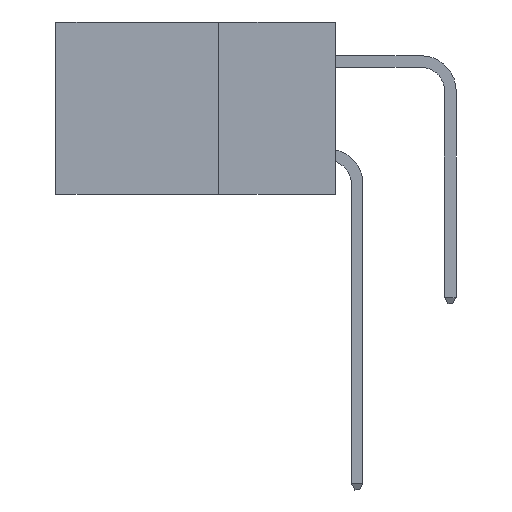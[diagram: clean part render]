
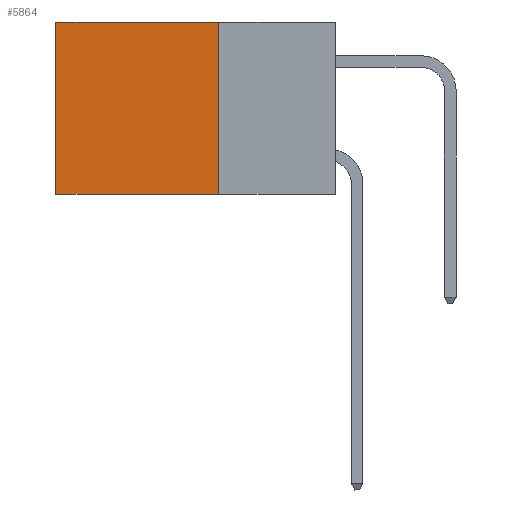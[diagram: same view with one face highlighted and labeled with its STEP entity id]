
A CAD part, left-side view. The second image highlights one B-rep face of the part: STEP entity #5864.
In plain terms, the highlighted planar face has unit normal (-1, 0, 0).
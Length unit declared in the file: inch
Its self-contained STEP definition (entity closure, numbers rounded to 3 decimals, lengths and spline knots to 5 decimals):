
#915 = VERTEX_POINT ( 'NONE', #24425 ) ;
#1086 = EDGE_CURVE ( 'NONE', #12607, #10471, #10237, .T. ) ;
#1834 = EDGE_CURVE ( 'NONE', #25764, #915, #17118, .T. ) ;
#2203 = DIRECTION ( 'NONE',  ( 0., 0., -1. ) ) ;
#3482 = CARTESIAN_POINT ( 'NONE',  ( 0.2875, 0.25, -0.37 ) ) ;
#3589 = VECTOR ( 'NONE', #23332, 39.37008 ) ;
#5864 = ADVANCED_FACE ( 'NONE', ( #30826 ), #12441, .F. ) ;
#6707 = DIRECTION ( 'NONE',  ( 0., 1., 0. ) ) ;
#7108 = VECTOR ( 'NONE', #23282, 39.37008 ) ;
#7812 = LINE ( 'NONE', #18786, #24448 ) ;
#9727 = CARTESIAN_POINT ( 'NONE',  ( 0.2875, 0.25, 0. ) ) ;
#9738 = CARTESIAN_POINT ( 'NONE',  ( 0.2875, 0.25, 0. ) ) ;
#9871 = DIRECTION ( 'NONE',  ( 1., 0., 0. ) ) ;
#10237 = LINE ( 'NONE', #9727, #17171 ) ;
#10471 = VERTEX_POINT ( 'NONE', #18738 ) ;
#12050 = AXIS2_PLACEMENT_3D ( 'NONE', #31842, #9871, #2203 ) ;
#12254 = ORIENTED_EDGE ( 'NONE', *, *, #13461, .F. ) ;
#12441 = PLANE ( 'NONE',  #12050 ) ;
#12607 = VERTEX_POINT ( 'NONE', #9738 ) ;
#13461 = EDGE_CURVE ( 'NONE', #10471, #915, #24474, .T. ) ;
#13725 = EDGE_CURVE ( 'NONE', #12607, #25764, #7812, .T. ) ;
#14568 = CARTESIAN_POINT ( 'NONE',  ( 0.2875, 0.6, 0. ) ) ;
#17118 = LINE ( 'NONE', #28404, #7108 ) ;
#17171 = VECTOR ( 'NONE', #29731, 39.37008 ) ;
#18738 = CARTESIAN_POINT ( 'NONE',  ( 0.2875, 0.25, -0.37 ) ) ;
#18786 = CARTESIAN_POINT ( 'NONE',  ( 0.2875, 0.25, 0. ) ) ;
#19856 = EDGE_LOOP ( 'NONE', ( #19935, #12254, #19969, #29141 ) ) ;
#19935 = ORIENTED_EDGE ( 'NONE', *, *, #1834, .T. ) ;
#19969 = ORIENTED_EDGE ( 'NONE', *, *, #1086, .F. ) ;
#23282 = DIRECTION ( 'NONE',  ( 0., 0., -1. ) ) ;
#23332 = DIRECTION ( 'NONE',  ( 0., 1., 0. ) ) ;
#24425 = CARTESIAN_POINT ( 'NONE',  ( 0.2875, 0.6, -0.37 ) ) ;
#24448 = VECTOR ( 'NONE', #6707, 39.37008 ) ;
#24474 = LINE ( 'NONE', #3482, #3589 ) ;
#25764 = VERTEX_POINT ( 'NONE', #14568 ) ;
#28404 = CARTESIAN_POINT ( 'NONE',  ( 0.2875, 0.6, 0. ) ) ;
#29141 = ORIENTED_EDGE ( 'NONE', *, *, #13725, .T. ) ;
#29731 = DIRECTION ( 'NONE',  ( 0., 0., -1. ) ) ;
#30826 = FACE_OUTER_BOUND ( 'NONE', #19856, .T. ) ;
#31842 = CARTESIAN_POINT ( 'NONE',  ( 0.2875, 0.25, 0. ) ) ;
